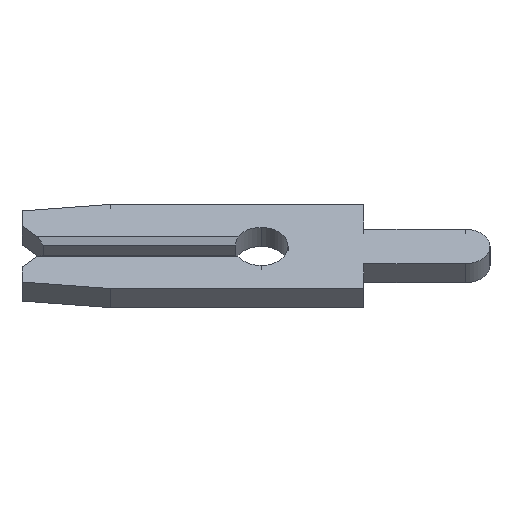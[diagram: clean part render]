
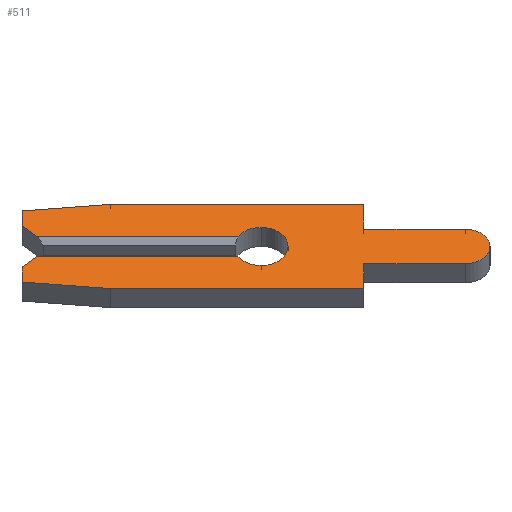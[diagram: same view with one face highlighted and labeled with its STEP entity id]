
A CAD part, left-side view. The second image highlights one B-rep face of the part: STEP entity #511.
In plain terms, the highlighted face is planar.
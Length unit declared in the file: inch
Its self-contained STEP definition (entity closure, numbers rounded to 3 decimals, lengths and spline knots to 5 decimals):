
#13 = DIRECTION ( 'NONE',  ( 0., -1., 0. ) ) ;
#16 = CARTESIAN_POINT ( 'NONE',  ( -0.013, 0.231, -0.028 ) ) ;
#19 = ORIENTED_EDGE ( 'NONE', *, *, #206, .F. ) ;
#23 = DIRECTION ( 'NONE',  ( 0., 0.995, 0.105 ) ) ;
#28 = ORIENTED_EDGE ( 'NONE', *, *, #760, .F. ) ;
#31 = AXIS2_PLACEMENT_3D ( 'NONE', #1018, #634, #1024 ) ;
#34 = DIRECTION ( 'NONE',  ( 0., 0.707, 0.707 ) ) ;
#36 = CARTESIAN_POINT ( 'NONE',  ( -0.013, 0.231, 0.04857 ) ) ;
#50 = LINE ( 'NONE', #903, #423 ) ;
#74 = EDGE_CURVE ( 'NONE', #740, #537, #50, .T. ) ;
#88 = ORIENTED_EDGE ( 'NONE', *, *, #1109, .F. ) ;
#90 = DIRECTION ( 'NONE',  ( 0., 0., -1. ) ) ;
#109 = CARTESIAN_POINT ( 'NONE',  ( -0.013, -0.099, -0.0235 ) ) ;
#119 = DIRECTION ( 'NONE',  ( 0., 1., 0. ) ) ;
#123 = EDGE_CURVE ( 'NONE', #942, #740, #721, .T. ) ;
#136 = CARTESIAN_POINT ( 'NONE',  ( -0.013, -0.099, -0.0575 ) ) ;
#148 = ORIENTED_EDGE ( 'NONE', *, *, #600, .F. ) ;
#152 = DIRECTION ( 'NONE',  ( 0., 0., -1. ) ) ;
#167 = FACE_OUTER_BOUND ( 'NONE', #1068, .T. ) ;
#186 = EDGE_CURVE ( 'NONE', #1159, #241, #530, .T. ) ;
#189 = VECTOR ( 'NONE', #1135, 39.37008 ) ;
#190 = CARTESIAN_POINT ( 'NONE',  ( -0.013, 0., 0. ) ) ;
#196 = CARTESIAN_POINT ( 'NONE',  ( -0.013, 0.216, -0.013 ) ) ;
#200 = ORIENTED_EDGE ( 'NONE', *, *, #257, .F. ) ;
#206 = EDGE_CURVE ( 'NONE', #424, #1159, #1175, .T. ) ;
#217 = VERTEX_POINT ( 'NONE', #621 ) ;
#226 = VECTOR ( 'NONE', #23, 39.37008 ) ;
#228 = VECTOR ( 'NONE', #1009, 39.37008 ) ;
#233 = CARTESIAN_POINT ( 'NONE',  ( -0.013, 0.231, -0.04857 ) ) ;
#238 = ORIENTED_EDGE ( 'NONE', *, *, #1180, .F. ) ;
#241 = VERTEX_POINT ( 'NONE', #1132 ) ;
#257 = EDGE_CURVE ( 'NONE', #454, #1107, #390, .T. ) ;
#261 = CARTESIAN_POINT ( 'NONE',  ( -0.013, 0.231, 0.04857 ) ) ;
#273 = VECTOR ( 'NONE', #455, 39.37008 ) ;
#276 = CARTESIAN_POINT ( 'NONE',  ( -0.013, -0.1975, 0.0235 ) ) ;
#290 = VERTEX_POINT ( 'NONE', #653 ) ;
#296 = EDGE_CURVE ( 'NONE', #1176, #290, #665, .T. ) ;
#300 = CIRCLE ( 'NONE', #604, 0.026 ) ;
#351 = DIRECTION ( 'NONE',  ( 0., -0.995, 0.105 ) ) ;
#353 = EDGE_CURVE ( 'NONE', #290, #1013, #766, .T. ) ;
#355 = CARTESIAN_POINT ( 'NONE',  ( -0.013, -0.099, -0.0575 ) ) ;
#374 = LINE ( 'NONE', #728, #226 ) ;
#381 = CARTESIAN_POINT ( 'NONE',  ( -0.013, 0.146, -0.0575 ) ) ;
#390 = CIRCLE ( 'NONE', #1074, 0.026 ) ;
#403 = ORIENTED_EDGE ( 'NONE', *, *, #1005, .F. ) ;
#423 = VECTOR ( 'NONE', #605, 39.37008 ) ;
#424 = VERTEX_POINT ( 'NONE', #276 ) ;
#426 = CARTESIAN_POINT ( 'NONE',  ( -0.013, 0.231, -0.028 ) ) ;
#431 = VERTEX_POINT ( 'NONE', #381 ) ;
#439 = LINE ( 'NONE', #569, #527 ) ;
#440 = CARTESIAN_POINT ( 'NONE',  ( -0.013, 0.146, 0.0575 ) ) ;
#445 = ORIENTED_EDGE ( 'NONE', *, *, #123, .F. ) ;
#454 = VERTEX_POINT ( 'NONE', #995 ) ;
#455 = DIRECTION ( 'NONE',  ( 0., -1., 0. ) ) ;
#470 = AXIS2_PLACEMENT_3D ( 'NONE', #190, #703, #90 ) ;
#493 = AXIS2_PLACEMENT_3D ( 'NONE', #738, #655, #152 ) ;
#511 = ADVANCED_FACE ( 'NONE', ( #167 ), #601, .F. ) ;
#517 = DIRECTION ( 'NONE',  ( -1., 0., 0. ) ) ;
#527 = VECTOR ( 'NONE', #673, 39.37008 ) ;
#530 = LINE ( 'NONE', #109, #1211 ) ;
#533 = EDGE_CURVE ( 'NONE', #647, #431, #1081, .T. ) ;
#537 = VERTEX_POINT ( 'NONE', #196 ) ;
#544 = LINE ( 'NONE', #551, #273 ) ;
#546 = CARTESIAN_POINT ( 'NONE',  ( -0.013, 0.231, 0.028 ) ) ;
#547 = VERTEX_POINT ( 'NONE', #796 ) ;
#551 = CARTESIAN_POINT ( 'NONE',  ( -0.013, 0.231, 0.013 ) ) ;
#554 = DIRECTION ( 'NONE',  ( 0., -1., 0. ) ) ;
#555 = CARTESIAN_POINT ( 'NONE',  ( -0.013, 0.2105, 0.0075 ) ) ;
#558 = CARTESIAN_POINT ( 'NONE',  ( -0.013, -0.099, 0.0575 ) ) ;
#569 = CARTESIAN_POINT ( 'NONE',  ( -0.013, 0., -0.013 ) ) ;
#575 = VECTOR ( 'NONE', #554, 39.37008 ) ;
#578 = CARTESIAN_POINT ( 'NONE',  ( -0.013, -0.099, 0.0575 ) ) ;
#595 = VERTEX_POINT ( 'NONE', #1111 ) ;
#600 = EDGE_CURVE ( 'NONE', #1096, #1176, #878, .T. ) ;
#601 = PLANE ( 'NONE',  #470 ) ;
#603 = ORIENTED_EDGE ( 'NONE', *, *, #941, .F. ) ;
#604 = AXIS2_PLACEMENT_3D ( 'NONE', #943, #517, #850 ) ;
#605 = DIRECTION ( 'NONE',  ( 0., -0.707, 0.707 ) ) ;
#616 = ORIENTED_EDGE ( 'NONE', *, *, #913, .F. ) ;
#621 = CARTESIAN_POINT ( 'NONE',  ( -0.013, -0.099, 0.0235 ) ) ;
#634 = DIRECTION ( 'NONE',  ( 1., 0., 0. ) ) ;
#644 = VECTOR ( 'NONE', #683, 39.37008 ) ;
#647 = VERTEX_POINT ( 'NONE', #136 ) ;
#653 = CARTESIAN_POINT ( 'NONE',  ( -0.013, 0.146, 0.0575 ) ) ;
#655 = DIRECTION ( 'NONE',  ( -1., 0., 0. ) ) ;
#658 = ORIENTED_EDGE ( 'NONE', *, *, #186, .F. ) ;
#659 = CARTESIAN_POINT ( 'NONE',  ( -0.013, -0.1975, -0.0235 ) ) ;
#663 = VECTOR ( 'NONE', #34, 39.37008 ) ;
#665 = LINE ( 'NONE', #36, #1288 ) ;
#666 = EDGE_CURVE ( 'NONE', #1107, #1040, #300, .T. ) ;
#673 = DIRECTION ( 'NONE',  ( 0., -1., 0. ) ) ;
#683 = DIRECTION ( 'NONE',  ( 0., 0., -1. ) ) ;
#703 = DIRECTION ( 'NONE',  ( 1., 0., 0. ) ) ;
#721 = LINE ( 'NONE', #16, #754 ) ;
#728 = CARTESIAN_POINT ( 'NONE',  ( -0.013, 0.231, -0.04857 ) ) ;
#738 = CARTESIAN_POINT ( 'NONE',  ( -0.013, 0., 0. ) ) ;
#740 = VERTEX_POINT ( 'NONE', #426 ) ;
#751 = CARTESIAN_POINT ( 'NONE',  ( -0.013, 0., 0.026 ) ) ;
#752 = CARTESIAN_POINT ( 'NONE',  ( -0.013, 0., 0. ) ) ;
#754 = VECTOR ( 'NONE', #827, 39.37008 ) ;
#756 = DIRECTION ( 'NONE',  ( 0., 0., -1. ) ) ;
#760 = EDGE_CURVE ( 'NONE', #431, #942, #374, .T. ) ;
#761 = ORIENTED_EDGE ( 'NONE', *, *, #296, .F. ) ;
#766 = LINE ( 'NONE', #440, #1232 ) ;
#788 = ORIENTED_EDGE ( 'NONE', *, *, #1029, .T. ) ;
#791 = EDGE_CURVE ( 'NONE', #547, #454, #1001, .T. ) ;
#793 = LINE ( 'NONE', #355, #860 ) ;
#796 = CARTESIAN_POINT ( 'NONE',  ( -0.013, 0.02252, -0.013 ) ) ;
#813 = CARTESIAN_POINT ( 'NONE',  ( -0.013, 0.231, 0.028 ) ) ;
#827 = DIRECTION ( 'NONE',  ( 0., 0., 1. ) ) ;
#831 = ORIENTED_EDGE ( 'NONE', *, *, #533, .F. ) ;
#844 = DIRECTION ( 'NONE',  ( 0., 0., -1. ) ) ;
#846 = LINE ( 'NONE', #555, #663 ) ;
#849 = CARTESIAN_POINT ( 'NONE',  ( -0.013, -0.099, 0.0235 ) ) ;
#850 = DIRECTION ( 'NONE',  ( 0., 0., -1. ) ) ;
#860 = VECTOR ( 'NONE', #756, 39.37008 ) ;
#878 = LINE ( 'NONE', #813, #189 ) ;
#903 = CARTESIAN_POINT ( 'NONE',  ( -0.013, 0.2105, -0.0075 ) ) ;
#910 = ORIENTED_EDGE ( 'NONE', *, *, #353, .F. ) ;
#913 = EDGE_CURVE ( 'NONE', #1013, #217, #1080, .T. ) ;
#941 = EDGE_CURVE ( 'NONE', #595, #1096, #846, .T. ) ;
#942 = VERTEX_POINT ( 'NONE', #233 ) ;
#943 = CARTESIAN_POINT ( 'NONE',  ( -0.013, 0., 0. ) ) ;
#945 = ORIENTED_EDGE ( 'NONE', *, *, #666, .F. ) ;
#956 = DIRECTION ( 'NONE',  ( -1., 0., 0. ) ) ;
#995 = CARTESIAN_POINT ( 'NONE',  ( -0.013, 0., -0.026 ) ) ;
#1001 = CIRCLE ( 'NONE', #493, 0.026 ) ;
#1005 = EDGE_CURVE ( 'NONE', #217, #424, #1142, .T. ) ;
#1009 = DIRECTION ( 'NONE',  ( 0., 1., 0. ) ) ;
#1013 = VERTEX_POINT ( 'NONE', #558 ) ;
#1018 = CARTESIAN_POINT ( 'NONE',  ( -0.013, -0.1975, 0. ) ) ;
#1024 = DIRECTION ( 'NONE',  ( 0., 0., 1. ) ) ;
#1029 = EDGE_CURVE ( 'NONE', #595, #1040, #544, .T. ) ;
#1040 = VERTEX_POINT ( 'NONE', #1057 ) ;
#1057 = CARTESIAN_POINT ( 'NONE',  ( -0.013, 0.02252, 0.013 ) ) ;
#1068 = EDGE_LOOP ( 'NONE', ( #788, #945, #200, #1199, #238, #1233, #445, #28, #831, #88, #658, #19, #403, #616, #910, #761, #148, #603 ) ) ;
#1074 = AXIS2_PLACEMENT_3D ( 'NONE', #752, #956, #844 ) ;
#1080 = LINE ( 'NONE', #578, #644 ) ;
#1081 = LINE ( 'NONE', #1093, #228 ) ;
#1093 = CARTESIAN_POINT ( 'NONE',  ( -0.013, 0.146, -0.0575 ) ) ;
#1096 = VERTEX_POINT ( 'NONE', #546 ) ;
#1107 = VERTEX_POINT ( 'NONE', #751 ) ;
#1109 = EDGE_CURVE ( 'NONE', #241, #647, #793, .T. ) ;
#1111 = CARTESIAN_POINT ( 'NONE',  ( -0.013, 0.216, 0.013 ) ) ;
#1132 = CARTESIAN_POINT ( 'NONE',  ( -0.013, -0.099, -0.0235 ) ) ;
#1135 = DIRECTION ( 'NONE',  ( 0., 0., 1. ) ) ;
#1142 = LINE ( 'NONE', #849, #575 ) ;
#1159 = VERTEX_POINT ( 'NONE', #659 ) ;
#1175 = CIRCLE ( 'NONE', #31, 0.0235 ) ;
#1176 = VERTEX_POINT ( 'NONE', #261 ) ;
#1180 = EDGE_CURVE ( 'NONE', #537, #547, #439, .T. ) ;
#1199 = ORIENTED_EDGE ( 'NONE', *, *, #791, .F. ) ;
#1211 = VECTOR ( 'NONE', #119, 39.37008 ) ;
#1232 = VECTOR ( 'NONE', #13, 39.37008 ) ;
#1233 = ORIENTED_EDGE ( 'NONE', *, *, #74, .F. ) ;
#1288 = VECTOR ( 'NONE', #351, 39.37008 ) ;
